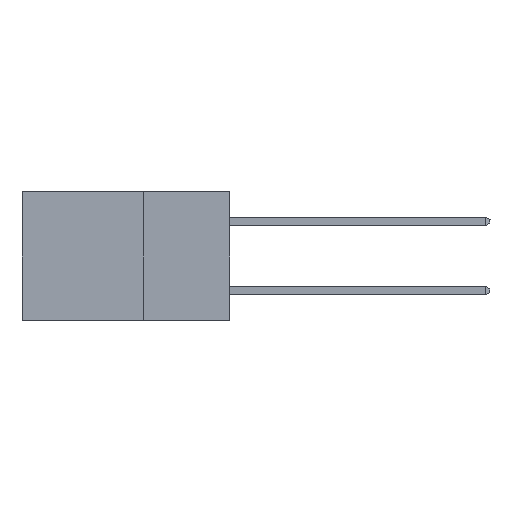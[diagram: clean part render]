
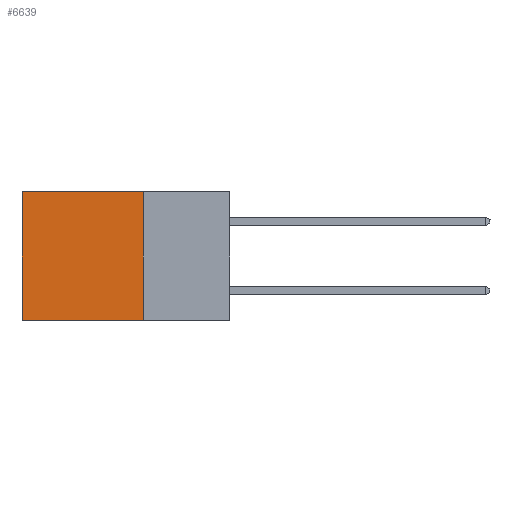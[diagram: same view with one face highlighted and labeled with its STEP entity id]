
A CAD part, left-side view. The second image highlights one B-rep face of the part: STEP entity #6639.
In plain terms, the highlighted planar face has unit normal (-1, 0, 0).
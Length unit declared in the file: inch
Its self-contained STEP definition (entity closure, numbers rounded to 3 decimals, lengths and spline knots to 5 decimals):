
#511 = EDGE_CURVE ( 'NONE', #10401, #15960, #16334, .T. ) ;
#750 = ORIENTED_EDGE ( 'NONE', *, *, #12724, .F. ) ;
#3119 = EDGE_LOOP ( 'NONE', ( #5133, #7320, #750, #12160 ) ) ;
#3976 = LINE ( 'NONE', #8123, #6256 ) ;
#4144 = CARTESIAN_POINT ( 'NONE',  ( 0.2615, 0.25, -0.37 ) ) ;
#4497 = AXIS2_PLACEMENT_3D ( 'NONE', #10717, #13553, #6575 ) ;
#5133 = ORIENTED_EDGE ( 'NONE', *, *, #10461, .T. ) ;
#5463 = CARTESIAN_POINT ( 'NONE',  ( 0.2615, 0.6, -0.37 ) ) ;
#6256 = VECTOR ( 'NONE', #13439, 39.37008 ) ;
#6575 = DIRECTION ( 'NONE',  ( 0., 0., -1. ) ) ;
#6639 = ADVANCED_FACE ( 'NONE', ( #16209 ), #16039, .F. ) ;
#6660 = VERTEX_POINT ( 'NONE', #16365 ) ;
#6971 = DIRECTION ( 'NONE',  ( 0., 1., 0. ) ) ;
#7320 = ORIENTED_EDGE ( 'NONE', *, *, #511, .F. ) ;
#7902 = CARTESIAN_POINT ( 'NONE',  ( 0.2615, 0.25, -0.37 ) ) ;
#8123 = CARTESIAN_POINT ( 'NONE',  ( 0.2615, 0.25, 0. ) ) ;
#8468 = VECTOR ( 'NONE', #11264, 39.37008 ) ;
#9674 = LINE ( 'NONE', #15336, #8468 ) ;
#10401 = VERTEX_POINT ( 'NONE', #7902 ) ;
#10461 = EDGE_CURVE ( 'NONE', #17381, #15960, #12322, .T. ) ;
#10717 = CARTESIAN_POINT ( 'NONE',  ( 0.2615, 0.25, -0.37 ) ) ;
#10826 = CARTESIAN_POINT ( 'NONE',  ( 0.2615, 0.6, -0.37 ) ) ;
#10911 = DIRECTION ( 'NONE',  ( 0., 0., -1. ) ) ;
#11264 = DIRECTION ( 'NONE',  ( 0., 0., -1. ) ) ;
#12160 = ORIENTED_EDGE ( 'NONE', *, *, #15347, .T. ) ;
#12322 = LINE ( 'NONE', #10826, #15220 ) ;
#12331 = CARTESIAN_POINT ( 'NONE',  ( 0.2615, 0.6, 0. ) ) ;
#12724 = EDGE_CURVE ( 'NONE', #6660, #10401, #9674, .T. ) ;
#13439 = DIRECTION ( 'NONE',  ( 0., 1., 0. ) ) ;
#13553 = DIRECTION ( 'NONE',  ( 1., 0., 0. ) ) ;
#14436 = VECTOR ( 'NONE', #6971, 39.37008 ) ;
#15220 = VECTOR ( 'NONE', #10911, 39.37008 ) ;
#15336 = CARTESIAN_POINT ( 'NONE',  ( 0.2615, 0.25, -0.37 ) ) ;
#15347 = EDGE_CURVE ( 'NONE', #6660, #17381, #3976, .T. ) ;
#15960 = VERTEX_POINT ( 'NONE', #5463 ) ;
#16039 = PLANE ( 'NONE',  #4497 ) ;
#16209 = FACE_OUTER_BOUND ( 'NONE', #3119, .T. ) ;
#16334 = LINE ( 'NONE', #4144, #14436 ) ;
#16365 = CARTESIAN_POINT ( 'NONE',  ( 0.2615, 0.25, 0. ) ) ;
#17381 = VERTEX_POINT ( 'NONE', #12331 ) ;
